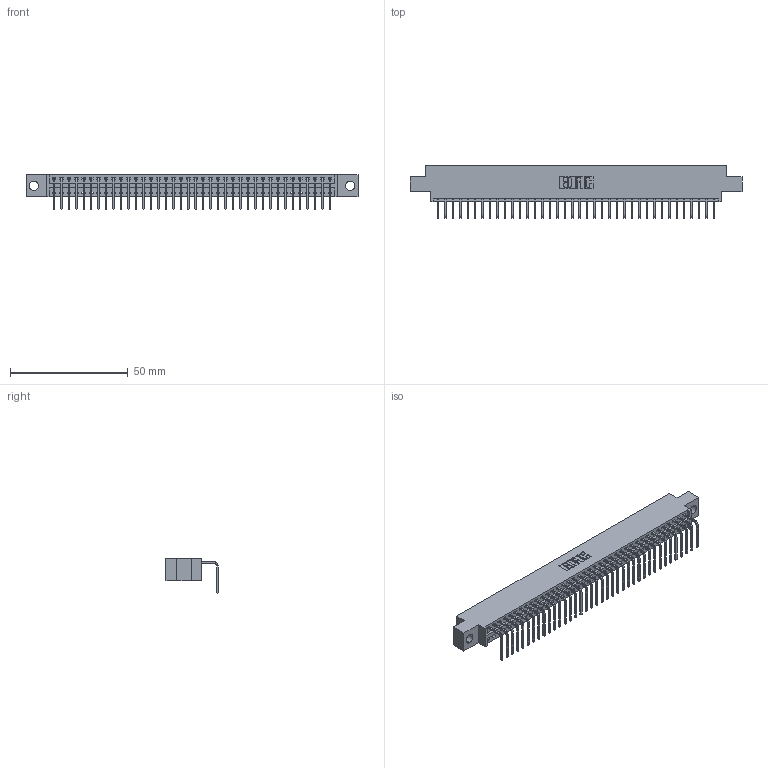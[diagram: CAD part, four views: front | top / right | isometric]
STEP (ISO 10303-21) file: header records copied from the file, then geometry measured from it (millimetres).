
FILE_DESCRIPTION (( 'STEP AP203' ), '1' );
FILE_NAME ('346-038-558-604.STEP', '2022-05-07T05:42:56', ( '' ), ( '' ), 'SwSTEP 2.0', 'SolidWorks 2020', '' );
FILE_SCHEMA (( 'CONFIG_CONTROL_DESIGN' ));
Length unit declared in the file: inch
Products named in the file (3): 346 Part_0.170 Offset - 0.156 Dia-TH; 345-292-001_558 Tail - 2; 346-038-558-604
Assembly tree (39 placements, depth 2):
  346-038-558-604
    346 Part_0.170 Offset - 0.156 Dia-TH
    345-292-001_558 Tail - 2  x38
Bounding box: 141.22 x 22.16 x 14.73 mm (x, y, z)
Volume: 13356.7 mm3; surface area: 17404 mm2
Topology: 39 solids, 39 shells, 2420 faces, 7293 edges, 4810 vertices
Faces by surface type: plane 1690, cylinder 730
Entity records: 24757 total; most frequent: CARTESIAN_POINT 4256, ORIENTED_EDGE 4226, DIRECTION 3757, EDGE_CURVE 2113, LINE 1829, VECTOR 1829, VERTEX_POINT 1406, AXIS2_PLACEMENT_3D 964
